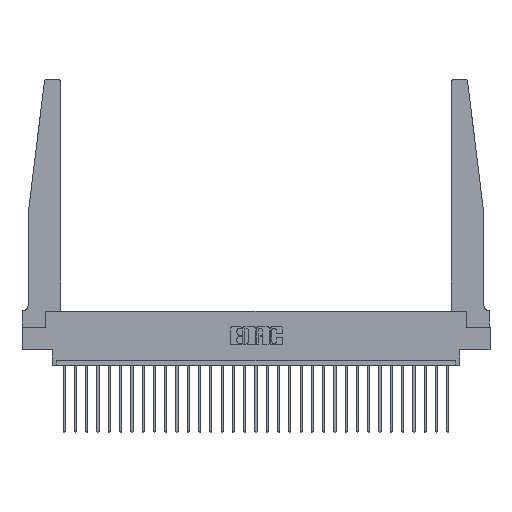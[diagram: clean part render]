
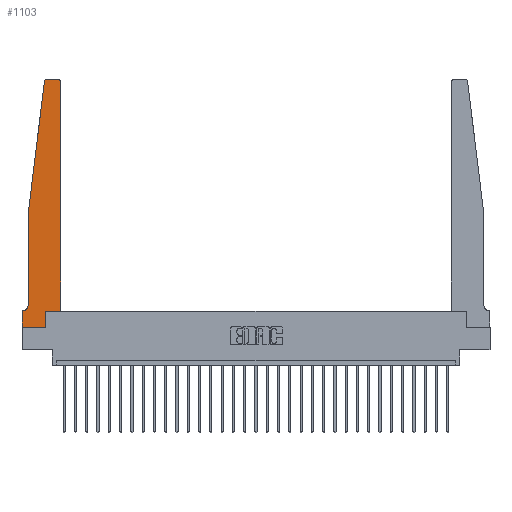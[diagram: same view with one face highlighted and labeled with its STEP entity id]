
A CAD part, top view. The second image highlights one B-rep face of the part: STEP entity #1103.
In plain terms, the highlighted planar face has unit normal (0, 0, 1).
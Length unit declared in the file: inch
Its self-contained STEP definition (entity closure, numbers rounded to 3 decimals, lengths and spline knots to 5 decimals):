
#70 = LINE ( 'NONE', #2046, #12064 ) ;
#179 = DIRECTION ( 'NONE',  ( 0., 1., 0. ) ) ;
#314 = ORIENTED_EDGE ( 'NONE', *, *, #6464, .T. ) ;
#427 = VECTOR ( 'NONE', #18381, 39.37008 ) ;
#699 = EDGE_CURVE ( 'NONE', #8942, #27550, #25559, .T. ) ;
#1103 = ADVANCED_FACE ( 'NONE', ( #4232 ), #1933, .T. ) ;
#1504 = VERTEX_POINT ( 'NONE', #5591 ) ;
#1832 = CARTESIAN_POINT ( 'NONE',  ( 0.065, 1.25, 0.37 ) ) ;
#1838 = VERTEX_POINT ( 'NONE', #19215 ) ;
#1933 = PLANE ( 'NONE',  #9417 ) ;
#2046 = CARTESIAN_POINT ( 'NONE',  ( 0.065, 1.25, 0.37 ) ) ;
#2053 = VERTEX_POINT ( 'NONE', #7655 ) ;
#2227 = DIRECTION ( 'NONE',  ( 1., 0., 0. ) ) ;
#2381 = CARTESIAN_POINT ( 'NONE',  ( 0.2605, 0.18, 0.37 ) ) ;
#2770 = DIRECTION ( 'NONE',  ( 0., 1., 0. ) ) ;
#2986 = LINE ( 'NONE', #22227, #6632 ) ;
#3035 = EDGE_CURVE ( 'NONE', #1838, #22211, #7464, .T. ) ;
#3046 = CARTESIAN_POINT ( 'NONE',  ( 0.27653, 2.75, 0.37 ) ) ;
#3280 = EDGE_CURVE ( 'NONE', #23134, #22992, #24403, .T. ) ;
#3575 = CARTESIAN_POINT ( 'NONE',  ( 0.015, 0.2375, 0.37 ) ) ;
#4217 = DIRECTION ( 'NONE',  ( 0., -1., 0. ) ) ;
#4232 = FACE_OUTER_BOUND ( 'NONE', #27307, .T. ) ;
#4378 = CARTESIAN_POINT ( 'NONE',  ( 0., 0., 0.37 ) ) ;
#4442 = CIRCLE ( 'NONE', #16476, 0.03 ) ;
#4836 = VERTEX_POINT ( 'NONE', #21749 ) ;
#5591 = CARTESIAN_POINT ( 'NONE',  ( 0.015, 0.1875, 0.37 ) ) ;
#5808 = VECTOR ( 'NONE', #23633, 39.37008 ) ;
#6464 = EDGE_CURVE ( 'NONE', #22211, #23134, #4442, .T. ) ;
#6632 = VECTOR ( 'NONE', #11924, 39.37008 ) ;
#7181 = VECTOR ( 'NONE', #179, 39.37008 ) ;
#7228 = AXIS2_PLACEMENT_3D ( 'NONE', #14719, #25835, #8991 ) ;
#7464 = LINE ( 'NONE', #26148, #23121 ) ;
#7655 = CARTESIAN_POINT ( 'NONE',  ( 0.2605, 0., 0.37 ) ) ;
#7728 = EDGE_CURVE ( 'NONE', #4836, #15273, #27058, .T. ) ;
#8125 = ORIENTED_EDGE ( 'NONE', *, *, #699, .T. ) ;
#8561 = DIRECTION ( 'NONE',  ( 0., 0., 1. ) ) ;
#8942 = VERTEX_POINT ( 'NONE', #24432 ) ;
#8991 = DIRECTION ( 'NONE',  ( 1., 0., 0. ) ) ;
#9205 = DIRECTION ( 'NONE',  ( 1., 0., 0. ) ) ;
#9417 = AXIS2_PLACEMENT_3D ( 'NONE', #16874, #8561, #2227 ) ;
#9433 = ORIENTED_EDGE ( 'NONE', *, *, #15395, .T. ) ;
#9818 = DIRECTION ( 'NONE',  ( 0., 0., -1. ) ) ;
#10124 = CARTESIAN_POINT ( 'NONE',  ( 0.065, 1.25, 0.37 ) ) ;
#10353 = ORIENTED_EDGE ( 'NONE', *, *, #7728, .T. ) ;
#10631 = DIRECTION ( 'NONE',  ( 0., -1., 0. ) ) ;
#10644 = CARTESIAN_POINT ( 'NONE',  ( 0., 0., 0.37 ) ) ;
#10949 = EDGE_CURVE ( 'NONE', #2053, #26739, #18536, .T. ) ;
#11716 = EDGE_CURVE ( 'NONE', #22992, #19695, #70, .T. ) ;
#11818 = ORIENTED_EDGE ( 'NONE', *, *, #10949, .T. ) ;
#11924 = DIRECTION ( 'NONE',  ( -1., 0., 0. ) ) ;
#12064 = VECTOR ( 'NONE', #4217, 39.37008 ) ;
#12682 = EDGE_CURVE ( 'NONE', #15273, #2053, #14521, .T. ) ;
#12859 = CARTESIAN_POINT ( 'NONE',  ( 0.2605, 0.18, 0.37 ) ) ;
#13051 = CARTESIAN_POINT ( 'NONE',  ( 0.425, 0.18, 0.37 ) ) ;
#13218 = EDGE_CURVE ( 'NONE', #27550, #1838, #23085, .T. ) ;
#13676 = VECTOR ( 'NONE', #9205, 39.37008 ) ;
#13677 = ORIENTED_EDGE ( 'NONE', *, *, #13218, .T. ) ;
#13932 = EDGE_CURVE ( 'NONE', #19695, #1504, #23378, .T. ) ;
#14521 = LINE ( 'NONE', #14944, #5808 ) ;
#14719 = CARTESIAN_POINT ( 'NONE',  ( 0.395, 2.72, 0.37 ) ) ;
#14937 = CARTESIAN_POINT ( 'NONE',  ( 0.065, 0.2375, 0.37 ) ) ;
#14944 = CARTESIAN_POINT ( 'NONE',  ( 0., 0., 0.37 ) ) ;
#15273 = VERTEX_POINT ( 'NONE', #10644 ) ;
#15395 = EDGE_CURVE ( 'NONE', #26739, #8942, #22956, .T. ) ;
#15571 = CARTESIAN_POINT ( 'NONE',  ( 0.425, 0.18, 0.37 ) ) ;
#15914 = VECTOR ( 'NONE', #2770, 39.37008 ) ;
#15963 = ORIENTED_EDGE ( 'NONE', *, *, #3280, .T. ) ;
#16476 = AXIS2_PLACEMENT_3D ( 'NONE', #22670, #24797, #22763 ) ;
#16874 = CARTESIAN_POINT ( 'NONE',  ( 0., 0.1875, 0.37 ) ) ;
#17773 = ORIENTED_EDGE ( 'NONE', *, *, #3035, .T. ) ;
#18381 = DIRECTION ( 'NONE',  ( -0.122, -0.992, 0. ) ) ;
#18536 = LINE ( 'NONE', #12859, #7181 ) ;
#19215 = CARTESIAN_POINT ( 'NONE',  ( 0.395, 2.75, 0.37 ) ) ;
#19695 = VERTEX_POINT ( 'NONE', #14937 ) ;
#20546 = ORIENTED_EDGE ( 'NONE', *, *, #13932, .T. ) ;
#21314 = ORIENTED_EDGE ( 'NONE', *, *, #11716, .T. ) ;
#21395 = CARTESIAN_POINT ( 'NONE',  ( 0.24675, 2.72367, 0.37 ) ) ;
#21749 = CARTESIAN_POINT ( 'NONE',  ( 0., 0.1875, 0.37 ) ) ;
#22211 = VERTEX_POINT ( 'NONE', #3046 ) ;
#22227 = CARTESIAN_POINT ( 'NONE',  ( 0.065, 0.1875, 0.37 ) ) ;
#22670 = CARTESIAN_POINT ( 'NONE',  ( 0.27653, 2.72, 0.37 ) ) ;
#22763 = DIRECTION ( 'NONE',  ( 1., 0., 0. ) ) ;
#22795 = AXIS2_PLACEMENT_3D ( 'NONE', #3575, #9818, #22811 ) ;
#22811 = DIRECTION ( 'NONE',  ( -1., 0., 0. ) ) ;
#22837 = ORIENTED_EDGE ( 'NONE', *, *, #12682, .T. ) ;
#22948 = CARTESIAN_POINT ( 'NONE',  ( 0.425, 2.72, 0.37 ) ) ;
#22956 = LINE ( 'NONE', #13051, #13676 ) ;
#22992 = VERTEX_POINT ( 'NONE', #1832 ) ;
#23085 = CIRCLE ( 'NONE', #7228, 0.03 ) ;
#23121 = VECTOR ( 'NONE', #24647, 39.37008 ) ;
#23134 = VERTEX_POINT ( 'NONE', #21395 ) ;
#23378 = CIRCLE ( 'NONE', #22795, 0.05 ) ;
#23633 = DIRECTION ( 'NONE',  ( 1., 0., 0. ) ) ;
#24351 = VECTOR ( 'NONE', #10631, 39.37008 ) ;
#24403 = LINE ( 'NONE', #10124, #427 ) ;
#24432 = CARTESIAN_POINT ( 'NONE',  ( 0.425, 0.18, 0.37 ) ) ;
#24647 = DIRECTION ( 'NONE',  ( -1., 0., 0. ) ) ;
#24797 = DIRECTION ( 'NONE',  ( 0., 0., 1. ) ) ;
#25032 = ORIENTED_EDGE ( 'NONE', *, *, #25434, .T. ) ;
#25434 = EDGE_CURVE ( 'NONE', #1504, #4836, #2986, .T. ) ;
#25559 = LINE ( 'NONE', #15571, #15914 ) ;
#25835 = DIRECTION ( 'NONE',  ( 0., 0., 1. ) ) ;
#26148 = CARTESIAN_POINT ( 'NONE',  ( 0.25, 2.75, 0.37 ) ) ;
#26739 = VERTEX_POINT ( 'NONE', #2381 ) ;
#27058 = LINE ( 'NONE', #4378, #24351 ) ;
#27307 = EDGE_LOOP ( 'NONE', ( #17773, #314, #15963, #21314, #20546, #25032, #10353, #22837, #11818, #9433, #8125, #13677 ) ) ;
#27550 = VERTEX_POINT ( 'NONE', #22948 ) ;
